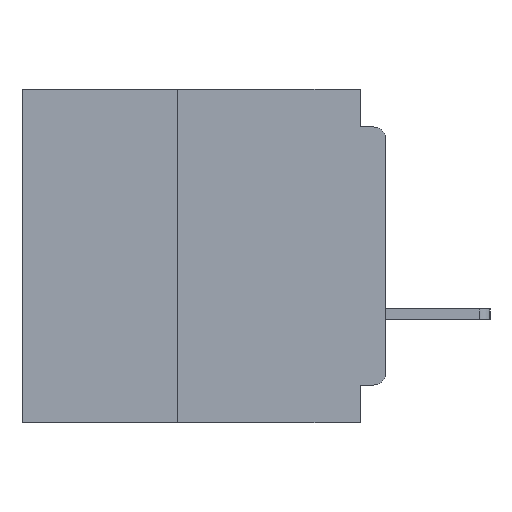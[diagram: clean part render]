
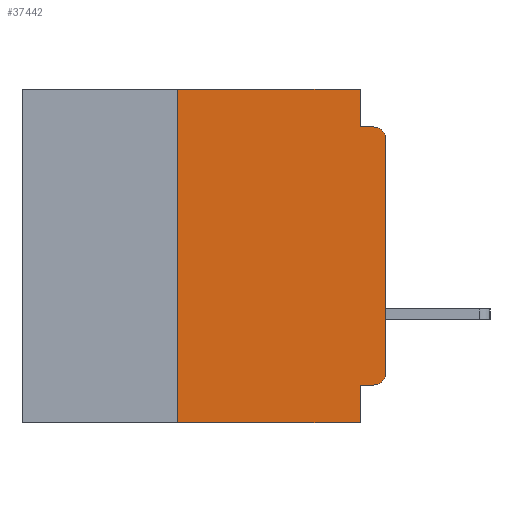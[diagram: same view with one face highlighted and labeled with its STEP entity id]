
A CAD part, left-side view. The second image highlights one B-rep face of the part: STEP entity #37442.
In plain terms, the highlighted planar face has unit normal (-1, 0, 0).
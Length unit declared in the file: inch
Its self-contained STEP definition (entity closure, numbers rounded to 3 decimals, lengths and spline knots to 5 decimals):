
#80 = CIRCLE ( 'NONE', #16945, 0.015 ) ;
#752 = EDGE_CURVE ( 'NONE', #22754, #37396, #2066, .T. ) ;
#1045 = EDGE_CURVE ( 'NONE', #8885, #34304, #30039, .T. ) ;
#1263 = CARTESIAN_POINT ( 'NONE',  ( 0., 0.25, -0.4 ) ) ;
#1494 = VECTOR ( 'NONE', #12296, 39.37008 ) ;
#2062 = EDGE_LOOP ( 'NONE', ( #19843, #30947, #23601, #7628, #8647, #11393, #25700, #14682, #7356, #21124 ) ) ;
#2066 = CIRCLE ( 'NONE', #23025, 0.015 ) ;
#2251 = LINE ( 'NONE', #6953, #32554 ) ;
#4017 = LINE ( 'NONE', #19226, #26511 ) ;
#5245 = VECTOR ( 'NONE', #21341, 39.37008 ) ;
#5340 = CARTESIAN_POINT ( 'NONE',  ( 0., 0.015, -0.045 ) ) ;
#5537 = VERTEX_POINT ( 'NONE', #34267 ) ;
#6447 = DIRECTION ( 'NONE',  ( 0., 1., 0. ) ) ;
#6953 = CARTESIAN_POINT ( 'NONE',  ( 0., 0.437, -0.4 ) ) ;
#6983 = VERTEX_POINT ( 'NONE', #15251 ) ;
#7221 = EDGE_CURVE ( 'NONE', #35467, #5537, #4017, .T. ) ;
#7356 = ORIENTED_EDGE ( 'NONE', *, *, #1045, .F. ) ;
#7560 = VERTEX_POINT ( 'NONE', #26944 ) ;
#7628 = ORIENTED_EDGE ( 'NONE', *, *, #7221, .F. ) ;
#8044 = LINE ( 'NONE', #26433, #22733 ) ;
#8483 = VECTOR ( 'NONE', #6447, 39.37008 ) ;
#8551 = DIRECTION ( 'NONE',  ( 0., 0., -1. ) ) ;
#8647 = ORIENTED_EDGE ( 'NONE', *, *, #33259, .F. ) ;
#8858 = DIRECTION ( 'NONE',  ( 0., -1., 0. ) ) ;
#8885 = VERTEX_POINT ( 'NONE', #12311 ) ;
#11161 = EDGE_CURVE ( 'NONE', #5537, #37396, #8044, .T. ) ;
#11393 = ORIENTED_EDGE ( 'NONE', *, *, #30136, .F. ) ;
#11678 = VECTOR ( 'NONE', #15851, 39.37008 ) ;
#12296 = DIRECTION ( 'NONE',  ( 0., 0., -1. ) ) ;
#12311 = CARTESIAN_POINT ( 'NONE',  ( 0., 0.015, -0.355 ) ) ;
#12592 = LINE ( 'NONE', #1263, #11678 ) ;
#12825 = CARTESIAN_POINT ( 'NONE',  ( 0., 0., -0.34 ) ) ;
#13036 = LINE ( 'NONE', #18377, #5245 ) ;
#14208 = VECTOR ( 'NONE', #14937, 39.37008 ) ;
#14242 = DIRECTION ( 'NONE',  ( -1., 0., 0. ) ) ;
#14682 = ORIENTED_EDGE ( 'NONE', *, *, #18115, .F. ) ;
#14912 = EDGE_CURVE ( 'NONE', #6983, #23852, #2251, .T. ) ;
#14937 = DIRECTION ( 'NONE',  ( 0., -1., 0. ) ) ;
#15251 = CARTESIAN_POINT ( 'NONE',  ( 0., 0.25, -0.4 ) ) ;
#15851 = DIRECTION ( 'NONE',  ( 0., 0., 1. ) ) ;
#16945 = AXIS2_PLACEMENT_3D ( 'NONE', #31859, #14242, #34779 ) ;
#17242 = PLANE ( 'NONE',  #25861 ) ;
#17975 = LINE ( 'NONE', #24108, #1494 ) ;
#18115 = EDGE_CURVE ( 'NONE', #34304, #23852, #17975, .T. ) ;
#18377 = CARTESIAN_POINT ( 'NONE',  ( 0., 0., 0. ) ) ;
#19226 = CARTESIAN_POINT ( 'NONE',  ( 0., 0.031, 0. ) ) ;
#19756 = CARTESIAN_POINT ( 'NONE',  ( 0., 0.031, -0.355 ) ) ;
#19843 = ORIENTED_EDGE ( 'NONE', *, *, #22585, .T. ) ;
#20194 = CARTESIAN_POINT ( 'NONE',  ( 0., 0.437, 0. ) ) ;
#21124 = ORIENTED_EDGE ( 'NONE', *, *, #36239, .T. ) ;
#21341 = DIRECTION ( 'NONE',  ( 0., 0., 1. ) ) ;
#21348 = DIRECTION ( 'NONE',  ( -1., 0., 0. ) ) ;
#21562 = CARTESIAN_POINT ( 'NONE',  ( 0., 0.015, -0.06 ) ) ;
#22156 = CARTESIAN_POINT ( 'NONE',  ( 0., 0.031, 0. ) ) ;
#22256 = CARTESIAN_POINT ( 'NONE',  ( 0., 0., -0.06 ) ) ;
#22585 = EDGE_CURVE ( 'NONE', #31385, #22754, #13036, .T. ) ;
#22733 = VECTOR ( 'NONE', #8858, 39.37008 ) ;
#22754 = VERTEX_POINT ( 'NONE', #22256 ) ;
#23025 = AXIS2_PLACEMENT_3D ( 'NONE', #21562, #21348, #30965 ) ;
#23601 = ORIENTED_EDGE ( 'NONE', *, *, #11161, .F. ) ;
#23852 = VERTEX_POINT ( 'NONE', #28383 ) ;
#24108 = CARTESIAN_POINT ( 'NONE',  ( 0., 0.031, -0.4 ) ) ;
#25309 = DIRECTION ( 'NONE',  ( 0., 0., -1. ) ) ;
#25700 = ORIENTED_EDGE ( 'NONE', *, *, #14912, .T. ) ;
#25861 = AXIS2_PLACEMENT_3D ( 'NONE', #20194, #26119, #8551 ) ;
#26119 = DIRECTION ( 'NONE',  ( 1., 0., 0. ) ) ;
#26433 = CARTESIAN_POINT ( 'NONE',  ( 0., 0., -0.045 ) ) ;
#26511 = VECTOR ( 'NONE', #25309, 39.37008 ) ;
#26944 = CARTESIAN_POINT ( 'NONE',  ( 0., 0.25, 0. ) ) ;
#27489 = DIRECTION ( 'NONE',  ( 0., -1., 0. ) ) ;
#28383 = CARTESIAN_POINT ( 'NONE',  ( 0., 0.031, -0.4 ) ) ;
#30039 = LINE ( 'NONE', #32843, #8483 ) ;
#30136 = EDGE_CURVE ( 'NONE', #6983, #7560, #12592, .T. ) ;
#30947 = ORIENTED_EDGE ( 'NONE', *, *, #752, .T. ) ;
#30965 = DIRECTION ( 'NONE',  ( 0., 0., -1. ) ) ;
#31385 = VERTEX_POINT ( 'NONE', #12825 ) ;
#31859 = CARTESIAN_POINT ( 'NONE',  ( 0., 0.015, -0.34 ) ) ;
#32553 = CARTESIAN_POINT ( 'NONE',  ( 0., 0.437, 0. ) ) ;
#32554 = VECTOR ( 'NONE', #27489, 39.37008 ) ;
#32843 = CARTESIAN_POINT ( 'NONE',  ( 0., 0., -0.355 ) ) ;
#33020 = FACE_OUTER_BOUND ( 'NONE', #2062, .T. ) ;
#33259 = EDGE_CURVE ( 'NONE', #7560, #35467, #36710, .T. ) ;
#34267 = CARTESIAN_POINT ( 'NONE',  ( 0., 0.031, -0.045 ) ) ;
#34304 = VERTEX_POINT ( 'NONE', #19756 ) ;
#34779 = DIRECTION ( 'NONE',  ( 0., 0., -1. ) ) ;
#35467 = VERTEX_POINT ( 'NONE', #22156 ) ;
#36239 = EDGE_CURVE ( 'NONE', #8885, #31385, #80, .T. ) ;
#36710 = LINE ( 'NONE', #32553, #14208 ) ;
#37396 = VERTEX_POINT ( 'NONE', #5340 ) ;
#37442 = ADVANCED_FACE ( 'NONE', ( #33020 ), #17242, .F. ) ;
